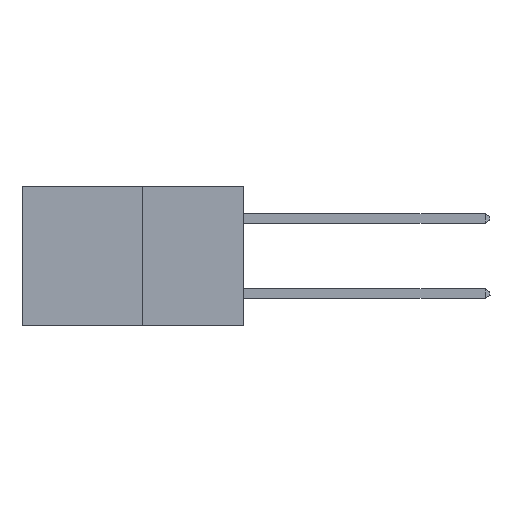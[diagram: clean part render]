
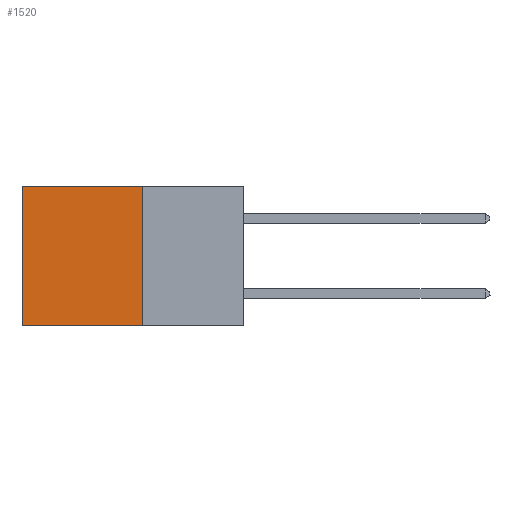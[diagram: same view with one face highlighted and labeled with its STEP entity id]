
A CAD part, left-side view. The second image highlights one B-rep face of the part: STEP entity #1520.
In plain terms, the highlighted planar face has unit normal (-1, 0, 0).
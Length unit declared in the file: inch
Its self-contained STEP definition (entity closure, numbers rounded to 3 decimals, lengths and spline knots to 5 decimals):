
#1393 = ORIENTED_EDGE ( 'NONE', *, *, #20233, .T. ) ;
#1520 = ADVANCED_FACE ( 'NONE', ( #10384 ), #16696, .F. ) ;
#3377 = VERTEX_POINT ( 'NONE', #20723 ) ;
#3680 = DIRECTION ( 'NONE',  ( 0., 1., 0. ) ) ;
#3868 = VECTOR ( 'NONE', #3680, 39.37008 ) ;
#4032 = DIRECTION ( 'NONE',  ( 0., 0., -1. ) ) ;
#4325 = CARTESIAN_POINT ( 'NONE',  ( 0.277, 0.59, -0.37 ) ) ;
#5719 = DIRECTION ( 'NONE',  ( 0., 1., 0. ) ) ;
#7386 = AXIS2_PLACEMENT_3D ( 'NONE', #19204, #19157, #17447 ) ;
#7907 = LINE ( 'NONE', #13795, #3868 ) ;
#9173 = CARTESIAN_POINT ( 'NONE',  ( 0.277, 0.27, -0.37 ) ) ;
#9455 = DIRECTION ( 'NONE',  ( 0., 0., -1. ) ) ;
#10384 = FACE_OUTER_BOUND ( 'NONE', #15299, .T. ) ;
#10549 = VECTOR ( 'NONE', #5719, 39.37008 ) ;
#10725 = EDGE_CURVE ( 'NONE', #18787, #3377, #15506, .T. ) ;
#10754 = VERTEX_POINT ( 'NONE', #14083 ) ;
#10786 = ORIENTED_EDGE ( 'NONE', *, *, #19675, .F. ) ;
#10823 = VECTOR ( 'NONE', #9455, 39.37008 ) ;
#11510 = ORIENTED_EDGE ( 'NONE', *, *, #21214, .T. ) ;
#12288 = ORIENTED_EDGE ( 'NONE', *, *, #10725, .F. ) ;
#13240 = CARTESIAN_POINT ( 'NONE',  ( 0.277, 0.59, 0. ) ) ;
#13447 = LINE ( 'NONE', #9173, #13966 ) ;
#13795 = CARTESIAN_POINT ( 'NONE',  ( 0.277, 0.27, 0. ) ) ;
#13966 = VECTOR ( 'NONE', #4032, 39.37008 ) ;
#14083 = CARTESIAN_POINT ( 'NONE',  ( 0.277, 0.27, 0. ) ) ;
#15229 = LINE ( 'NONE', #4325, #10823 ) ;
#15299 = EDGE_LOOP ( 'NONE', ( #1393, #12288, #10786, #11510 ) ) ;
#15506 = LINE ( 'NONE', #20734, #10549 ) ;
#16696 = PLANE ( 'NONE',  #7386 ) ;
#17447 = DIRECTION ( 'NONE',  ( 0., 0., -1. ) ) ;
#18769 = CARTESIAN_POINT ( 'NONE',  ( 0.277, 0.27, -0.37 ) ) ;
#18787 = VERTEX_POINT ( 'NONE', #18769 ) ;
#19157 = DIRECTION ( 'NONE',  ( 1., 0., 0. ) ) ;
#19204 = CARTESIAN_POINT ( 'NONE',  ( 0.277, 0.27, -0.37 ) ) ;
#19675 = EDGE_CURVE ( 'NONE', #10754, #18787, #13447, .T. ) ;
#20233 = EDGE_CURVE ( 'NONE', #20438, #3377, #15229, .T. ) ;
#20438 = VERTEX_POINT ( 'NONE', #13240 ) ;
#20723 = CARTESIAN_POINT ( 'NONE',  ( 0.277, 0.59, -0.37 ) ) ;
#20734 = CARTESIAN_POINT ( 'NONE',  ( 0.277, 0.27, -0.37 ) ) ;
#21214 = EDGE_CURVE ( 'NONE', #10754, #20438, #7907, .T. ) ;
